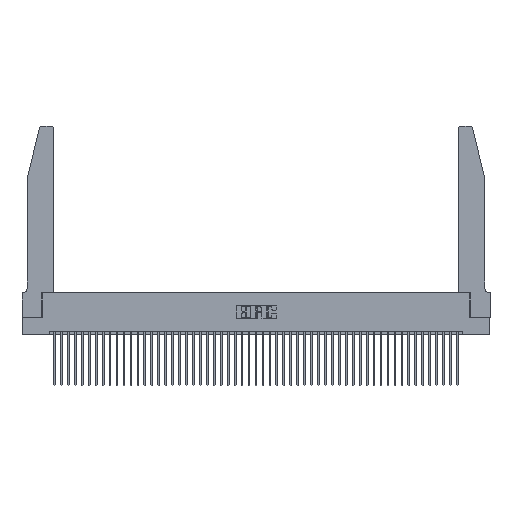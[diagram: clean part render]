
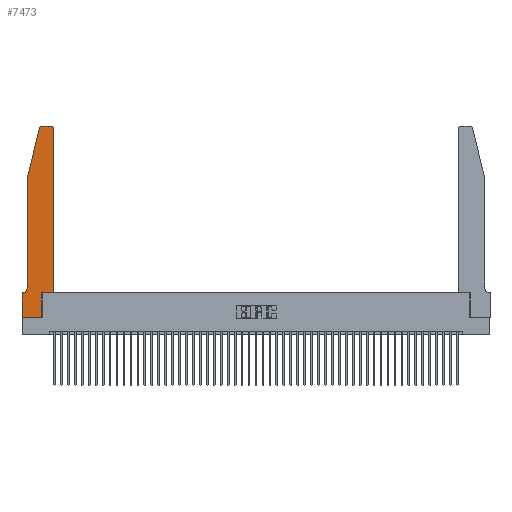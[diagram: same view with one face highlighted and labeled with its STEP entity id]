
A CAD part, top view. The second image highlights one B-rep face of the part: STEP entity #7473.
In plain terms, the highlighted planar face has unit normal (0, 0, 1).
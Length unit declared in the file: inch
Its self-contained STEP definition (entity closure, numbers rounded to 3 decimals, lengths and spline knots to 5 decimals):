
#1239 = CARTESIAN_POINT ( 'NONE',  ( 0.0055, 0.42, 0.37 ) ) ;
#1716 = DIRECTION ( 'NONE',  ( 1., 0., 0. ) ) ;
#2700 = LINE ( 'NONE', #20200, #8663 ) ;
#2736 = EDGE_CURVE ( 'NONE', #28368, #36038, #39559, .T. ) ;
#3062 = CARTESIAN_POINT ( 'NONE',  ( 0.4505, 0.35, 0.37 ) ) ;
#3359 = CARTESIAN_POINT ( 'NONE',  ( 0.0755, 0.42, 0.37 ) ) ;
#4268 = CARTESIAN_POINT ( 'NONE',  ( 0.0755, 2., 0.37 ) ) ;
#4329 = CARTESIAN_POINT ( 'NONE',  ( 0.25487, 2.72718, 0.37 ) ) ;
#4733 = VECTOR ( 'NONE', #36643, 39.37008 ) ;
#4829 = VERTEX_POINT ( 'NONE', #7476 ) ;
#5030 = DIRECTION ( 'NONE',  ( 1., 0., 0. ) ) ;
#6488 = AXIS2_PLACEMENT_3D ( 'NONE', #47727, #40362, #33771 ) ;
#6546 = DIRECTION ( 'NONE',  ( -1., 0., 0. ) ) ;
#7220 = PLANE ( 'NONE',  #6488 ) ;
#7473 = ADVANCED_FACE ( 'NONE', ( #16717 ), #7220, .T. ) ;
#7476 = CARTESIAN_POINT ( 'NONE',  ( 0., 0., 0.37 ) ) ;
#7725 = CARTESIAN_POINT ( 'NONE',  ( 0.0755, 0.35, 0.37 ) ) ;
#8064 = EDGE_CURVE ( 'NONE', #25399, #4829, #12692, .T. ) ;
#8145 = ORIENTED_EDGE ( 'NONE', *, *, #23855, .T. ) ;
#8355 = EDGE_CURVE ( 'NONE', #33906, #33952, #20294, .T. ) ;
#8663 = VECTOR ( 'NONE', #6546, 39.37008 ) ;
#8745 = CIRCLE ( 'NONE', #27432, 0.03 ) ;
#9294 = ORIENTED_EDGE ( 'NONE', *, *, #20705, .T. ) ;
#9646 = LINE ( 'NONE', #25943, #38539 ) ;
#9970 = VERTEX_POINT ( 'NONE', #47882 ) ;
#10004 = CARTESIAN_POINT ( 'NONE',  ( 0.2865, 0., 0.37 ) ) ;
#11108 = ORIENTED_EDGE ( 'NONE', *, *, #36161, .T. ) ;
#11521 = VECTOR ( 'NONE', #29252, 39.37008 ) ;
#11882 = CARTESIAN_POINT ( 'NONE',  ( 0.284, 2.75, 0.37 ) ) ;
#12131 = ORIENTED_EDGE ( 'NONE', *, *, #30272, .T. ) ;
#12692 = LINE ( 'NONE', #19059, #35144 ) ;
#13104 = DIRECTION ( 'NONE',  ( -1., 0., 0. ) ) ;
#13853 = DIRECTION ( 'NONE',  ( 0., -1., 0. ) ) ;
#15236 = CARTESIAN_POINT ( 'NONE',  ( 0.0055, 0.35, 0.37 ) ) ;
#15719 = VERTEX_POINT ( 'NONE', #4268 ) ;
#15942 = ORIENTED_EDGE ( 'NONE', *, *, #16792, .T. ) ;
#16717 = FACE_OUTER_BOUND ( 'NONE', #45168, .T. ) ;
#16792 = EDGE_CURVE ( 'NONE', #4829, #28368, #34224, .T. ) ;
#17869 = ORIENTED_EDGE ( 'NONE', *, *, #2736, .T. ) ;
#18273 = CARTESIAN_POINT ( 'NONE',  ( 0.2865, 0.35, 0.37 ) ) ;
#18685 = EDGE_CURVE ( 'NONE', #41289, #9970, #8745, .T. ) ;
#18853 = DIRECTION ( 'NONE',  ( -0.239, -0.971, 0. ) ) ;
#18940 = DIRECTION ( 'NONE',  ( 1., 0., 0. ) ) ;
#19059 = CARTESIAN_POINT ( 'NONE',  ( 0., 0., 0.37 ) ) ;
#19239 = DIRECTION ( 'NONE',  ( -1., 0., 0. ) ) ;
#20031 = ORIENTED_EDGE ( 'NONE', *, *, #20282, .T. ) ;
#20058 = VERTEX_POINT ( 'NONE', #11882 ) ;
#20200 = CARTESIAN_POINT ( 'NONE',  ( 0.2605, 2.75, 0.37 ) ) ;
#20282 = EDGE_CURVE ( 'NONE', #15719, #33906, #28623, .T. ) ;
#20294 = CIRCLE ( 'NONE', #30520, 0.07 ) ;
#20705 = EDGE_CURVE ( 'NONE', #20058, #28709, #29735, .T. ) ;
#22486 = DIRECTION ( 'NONE',  ( 0., -1., 0. ) ) ;
#22607 = VERTEX_POINT ( 'NONE', #3062 ) ;
#22686 = LINE ( 'NONE', #28778, #11521 ) ;
#23812 = DIRECTION ( 'NONE',  ( 0., 0., -1. ) ) ;
#23855 = EDGE_CURVE ( 'NONE', #9970, #20058, #2700, .T. ) ;
#23973 = CARTESIAN_POINT ( 'NONE',  ( 0.284, 2.72, 0.37 ) ) ;
#23991 = AXIS2_PLACEMENT_3D ( 'NONE', #23973, #27496, #1716 ) ;
#24908 = CARTESIAN_POINT ( 'NONE',  ( 0.2865, 0.35, 0.37 ) ) ;
#25399 = VERTEX_POINT ( 'NONE', #34099 ) ;
#25943 = CARTESIAN_POINT ( 'NONE',  ( 0.0755, 2., 0.37 ) ) ;
#26755 = ORIENTED_EDGE ( 'NONE', *, *, #8064, .T. ) ;
#27432 = AXIS2_PLACEMENT_3D ( 'NONE', #33478, #44797, #18940 ) ;
#27496 = DIRECTION ( 'NONE',  ( 0., 0., 1. ) ) ;
#27953 = CARTESIAN_POINT ( 'NONE',  ( 0.4505, 0.35, 0.37 ) ) ;
#28368 = VERTEX_POINT ( 'NONE', #10004 ) ;
#28623 = LINE ( 'NONE', #47780, #30347 ) ;
#28709 = VERTEX_POINT ( 'NONE', #4329 ) ;
#28778 = CARTESIAN_POINT ( 'NONE',  ( 0.4505, 0.35, 0.37 ) ) ;
#29252 = DIRECTION ( 'NONE',  ( 0., 1., 0. ) ) ;
#29735 = CIRCLE ( 'NONE', #23991, 0.03 ) ;
#30272 = EDGE_CURVE ( 'NONE', #36038, #22607, #45192, .T. ) ;
#30347 = VECTOR ( 'NONE', #13853, 39.37008 ) ;
#30520 = AXIS2_PLACEMENT_3D ( 'NONE', #1239, #23812, #13104 ) ;
#32414 = ORIENTED_EDGE ( 'NONE', *, *, #8355, .T. ) ;
#33478 = CARTESIAN_POINT ( 'NONE',  ( 0.4205, 2.72, 0.37 ) ) ;
#33771 = DIRECTION ( 'NONE',  ( 1., 0., 0. ) ) ;
#33906 = VERTEX_POINT ( 'NONE', #3359 ) ;
#33952 = VERTEX_POINT ( 'NONE', #15236 ) ;
#34099 = CARTESIAN_POINT ( 'NONE',  ( 0., 0.35, 0.37 ) ) ;
#34224 = LINE ( 'NONE', #39810, #41858 ) ;
#35144 = VECTOR ( 'NONE', #22486, 39.37008 ) ;
#35218 = VECTOR ( 'NONE', #5030, 39.37008 ) ;
#36038 = VERTEX_POINT ( 'NONE', #18273 ) ;
#36161 = EDGE_CURVE ( 'NONE', #33952, #25399, #42311, .T. ) ;
#36391 = ORIENTED_EDGE ( 'NONE', *, *, #42268, .T. ) ;
#36643 = DIRECTION ( 'NONE',  ( 0., 1., 0. ) ) ;
#37242 = EDGE_CURVE ( 'NONE', #22607, #41289, #22686, .T. ) ;
#38261 = ORIENTED_EDGE ( 'NONE', *, *, #18685, .T. ) ;
#38539 = VECTOR ( 'NONE', #18853, 39.37008 ) ;
#39323 = DIRECTION ( 'NONE',  ( 1., 0., 0. ) ) ;
#39559 = LINE ( 'NONE', #24908, #4733 ) ;
#39810 = CARTESIAN_POINT ( 'NONE',  ( 0., 0., 0.37 ) ) ;
#40362 = DIRECTION ( 'NONE',  ( 0., 0., 1. ) ) ;
#41060 = ORIENTED_EDGE ( 'NONE', *, *, #37242, .T. ) ;
#41289 = VERTEX_POINT ( 'NONE', #44698 ) ;
#41858 = VECTOR ( 'NONE', #39323, 39.37008 ) ;
#42268 = EDGE_CURVE ( 'NONE', #28709, #15719, #9646, .T. ) ;
#42311 = LINE ( 'NONE', #7725, #45838 ) ;
#44698 = CARTESIAN_POINT ( 'NONE',  ( 0.4505, 2.72, 0.37 ) ) ;
#44797 = DIRECTION ( 'NONE',  ( 0., 0., 1. ) ) ;
#45168 = EDGE_LOOP ( 'NONE', ( #8145, #9294, #36391, #20031, #32414, #11108, #26755, #15942, #17869, #12131, #41060, #38261 ) ) ;
#45192 = LINE ( 'NONE', #27953, #35218 ) ;
#45838 = VECTOR ( 'NONE', #19239, 39.37008 ) ;
#47727 = CARTESIAN_POINT ( 'NONE',  ( 0., 0.35, 0.37 ) ) ;
#47780 = CARTESIAN_POINT ( 'NONE',  ( 0.0755, 2., 0.37 ) ) ;
#47882 = CARTESIAN_POINT ( 'NONE',  ( 0.4205, 2.75, 0.37 ) ) ;
